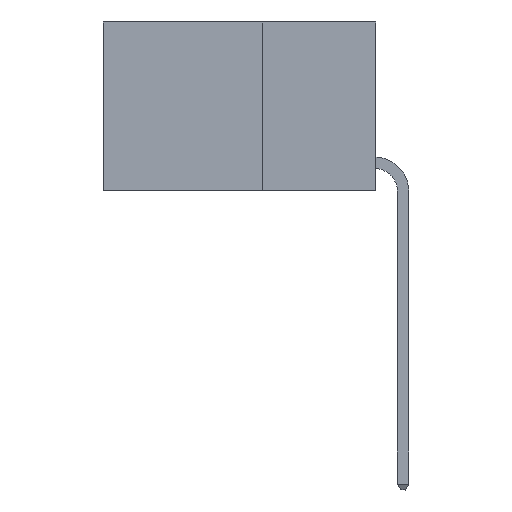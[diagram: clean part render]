
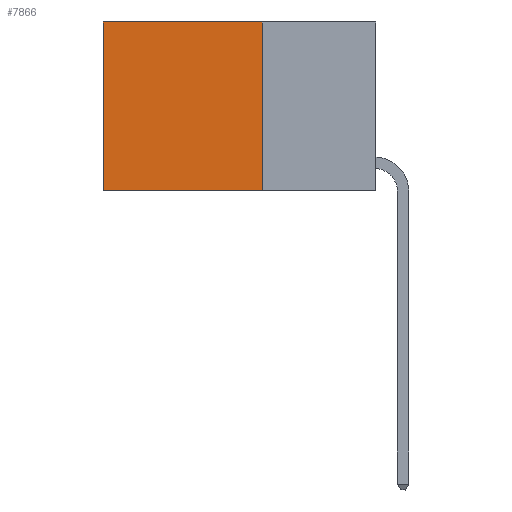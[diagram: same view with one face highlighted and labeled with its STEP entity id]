
A CAD part, left-side view. The second image highlights one B-rep face of the part: STEP entity #7866.
In plain terms, the highlighted planar face has unit normal (-1, 0, 0).
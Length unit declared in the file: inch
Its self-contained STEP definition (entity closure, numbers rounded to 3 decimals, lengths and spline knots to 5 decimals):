
#1341 = ORIENTED_EDGE ( 'NONE', *, *, #17695, .F. ) ;
#1371 = CARTESIAN_POINT ( 'NONE',  ( 0.2625, 0.25, 0. ) ) ;
#1949 = LINE ( 'NONE', #23452, #20170 ) ;
#2838 = LINE ( 'NONE', #16437, #16336 ) ;
#2958 = DIRECTION ( 'NONE',  ( 0., 1., 0. ) ) ;
#3040 = DIRECTION ( 'NONE',  ( 0., 0., -1. ) ) ;
#3869 = ORIENTED_EDGE ( 'NONE', *, *, #5863, .F. ) ;
#4520 = LINE ( 'NONE', #21799, #6845 ) ;
#5345 = DIRECTION ( 'NONE',  ( 1., 0., 0. ) ) ;
#5863 = EDGE_CURVE ( 'NONE', #10836, #7488, #1949, .T. ) ;
#6845 = VECTOR ( 'NONE', #2958, 39.37008 ) ;
#7488 = VERTEX_POINT ( 'NONE', #21228 ) ;
#7866 = ADVANCED_FACE ( 'NONE', ( #20931 ), #21194, .F. ) ;
#8484 = LINE ( 'NONE', #12006, #18154 ) ;
#8633 = EDGE_CURVE ( 'NONE', #23329, #13721, #4520, .T. ) ;
#8732 = CARTESIAN_POINT ( 'NONE',  ( 0.2625, 0.25, -0.37 ) ) ;
#10836 = VERTEX_POINT ( 'NONE', #8732 ) ;
#11232 = CARTESIAN_POINT ( 'NONE',  ( 0.2625, 0.6, 0. ) ) ;
#12006 = CARTESIAN_POINT ( 'NONE',  ( 0.2625, 0.6, 0. ) ) ;
#12488 = EDGE_LOOP ( 'NONE', ( #12892, #3869, #1341, #22947 ) ) ;
#12796 = DIRECTION ( 'NONE',  ( 0., 0., -1. ) ) ;
#12892 = ORIENTED_EDGE ( 'NONE', *, *, #23446, .T. ) ;
#13721 = VERTEX_POINT ( 'NONE', #11232 ) ;
#16030 = DIRECTION ( 'NONE',  ( 0., 0., -1. ) ) ;
#16336 = VECTOR ( 'NONE', #12796, 39.37008 ) ;
#16437 = CARTESIAN_POINT ( 'NONE',  ( 0.2625, 0.25, 0. ) ) ;
#17695 = EDGE_CURVE ( 'NONE', #23329, #10836, #2838, .T. ) ;
#18154 = VECTOR ( 'NONE', #16030, 39.37008 ) ;
#19416 = DIRECTION ( 'NONE',  ( 0., 1., 0. ) ) ;
#20170 = VECTOR ( 'NONE', #19416, 39.37008 ) ;
#20931 = FACE_OUTER_BOUND ( 'NONE', #12488, .T. ) ;
#21194 = PLANE ( 'NONE',  #21312 ) ;
#21228 = CARTESIAN_POINT ( 'NONE',  ( 0.2625, 0.6, -0.37 ) ) ;
#21312 = AXIS2_PLACEMENT_3D ( 'NONE', #1371, #5345, #3040 ) ;
#21799 = CARTESIAN_POINT ( 'NONE',  ( 0.2625, 0.25, 0. ) ) ;
#22947 = ORIENTED_EDGE ( 'NONE', *, *, #8633, .T. ) ;
#23329 = VERTEX_POINT ( 'NONE', #23416 ) ;
#23416 = CARTESIAN_POINT ( 'NONE',  ( 0.2625, 0.25, 0. ) ) ;
#23446 = EDGE_CURVE ( 'NONE', #13721, #7488, #8484, .T. ) ;
#23452 = CARTESIAN_POINT ( 'NONE',  ( 0.2625, 0.25, -0.37 ) ) ;
